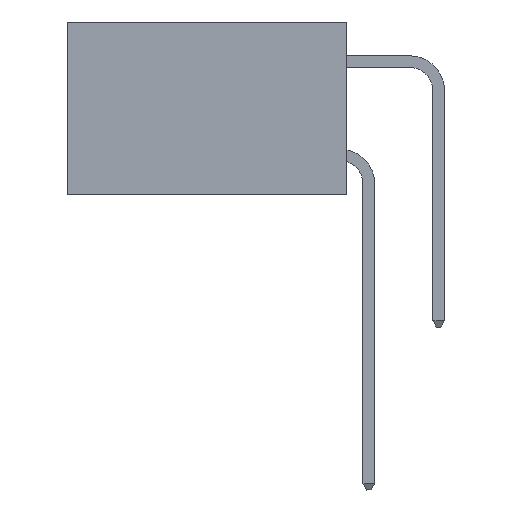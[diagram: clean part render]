
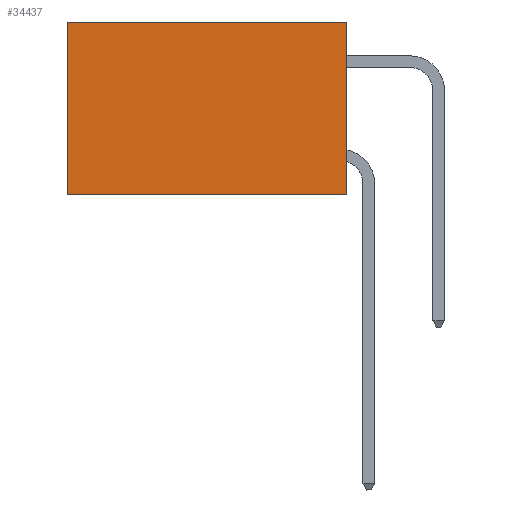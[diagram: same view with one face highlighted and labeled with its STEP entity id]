
A CAD part, left-side view. The second image highlights one B-rep face of the part: STEP entity #34437.
In plain terms, the highlighted planar face has unit normal (-1, 0, 0).
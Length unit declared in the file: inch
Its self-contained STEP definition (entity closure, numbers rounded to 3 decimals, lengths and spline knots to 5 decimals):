
#278 = CARTESIAN_POINT ( 'NONE',  ( 0.2875, 0., -0.37 ) ) ;
#496 = LINE ( 'NONE', #4475, #22235 ) ;
#831 = ORIENTED_EDGE ( 'NONE', *, *, #11747, .T. ) ;
#1069 = ORIENTED_EDGE ( 'NONE', *, *, #24761, .T. ) ;
#2542 = DIRECTION ( 'NONE',  ( 0., 0., -1. ) ) ;
#2680 = CARTESIAN_POINT ( 'NONE',  ( 0.2875, 0.6, -0.37 ) ) ;
#4475 = CARTESIAN_POINT ( 'NONE',  ( 0.2875, 0., -0.37 ) ) ;
#5308 = VERTEX_POINT ( 'NONE', #2680 ) ;
#8672 = VECTOR ( 'NONE', #29679, 39.37008 ) ;
#9227 = DIRECTION ( 'NONE',  ( 0., 0., -1. ) ) ;
#11151 = VECTOR ( 'NONE', #13303, 39.37008 ) ;
#11747 = EDGE_CURVE ( 'NONE', #34864, #5308, #12349, .T. ) ;
#12349 = LINE ( 'NONE', #34914, #25784 ) ;
#13303 = DIRECTION ( 'NONE',  ( 0., 0., -1. ) ) ;
#13318 = CARTESIAN_POINT ( 'NONE',  ( 0.2875, 0., 0. ) ) ;
#15743 = EDGE_LOOP ( 'NONE', ( #831, #27595, #32344, #1069 ) ) ;
#19278 = EDGE_CURVE ( 'NONE', #34130, #5308, #496, .T. ) ;
#19957 = PLANE ( 'NONE',  #34446 ) ;
#20705 = DIRECTION ( 'NONE',  ( 0., 1., 0. ) ) ;
#21366 = VERTEX_POINT ( 'NONE', #13318 ) ;
#21434 = CARTESIAN_POINT ( 'NONE',  ( 0.2875, 0.6, 0. ) ) ;
#22235 = VECTOR ( 'NONE', #20705, 39.37008 ) ;
#22635 = CARTESIAN_POINT ( 'NONE',  ( 0.2875, 0., 0. ) ) ;
#24761 = EDGE_CURVE ( 'NONE', #21366, #34864, #29237, .T. ) ;
#25347 = DIRECTION ( 'NONE',  ( 1., 0., 0. ) ) ;
#25784 = VECTOR ( 'NONE', #2542, 39.37008 ) ;
#26043 = EDGE_CURVE ( 'NONE', #21366, #34130, #31641, .T. ) ;
#27003 = CARTESIAN_POINT ( 'NONE',  ( 0.2875, 0., 0. ) ) ;
#27595 = ORIENTED_EDGE ( 'NONE', *, *, #19278, .F. ) ;
#29237 = LINE ( 'NONE', #27003, #8672 ) ;
#29679 = DIRECTION ( 'NONE',  ( 0., 1., 0. ) ) ;
#31641 = LINE ( 'NONE', #31958, #11151 ) ;
#31958 = CARTESIAN_POINT ( 'NONE',  ( 0.2875, 0., 0. ) ) ;
#32344 = ORIENTED_EDGE ( 'NONE', *, *, #26043, .F. ) ;
#34130 = VERTEX_POINT ( 'NONE', #278 ) ;
#34437 = ADVANCED_FACE ( 'NONE', ( #34818 ), #19957, .F. ) ;
#34446 = AXIS2_PLACEMENT_3D ( 'NONE', #22635, #25347, #9227 ) ;
#34818 = FACE_OUTER_BOUND ( 'NONE', #15743, .T. ) ;
#34864 = VERTEX_POINT ( 'NONE', #21434 ) ;
#34914 = CARTESIAN_POINT ( 'NONE',  ( 0.2875, 0.6, 0. ) ) ;
